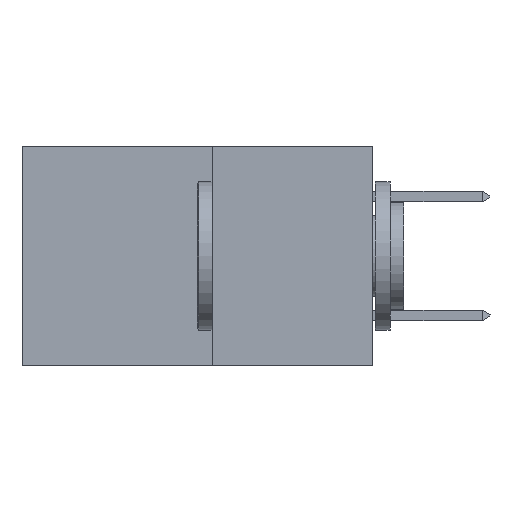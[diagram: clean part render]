
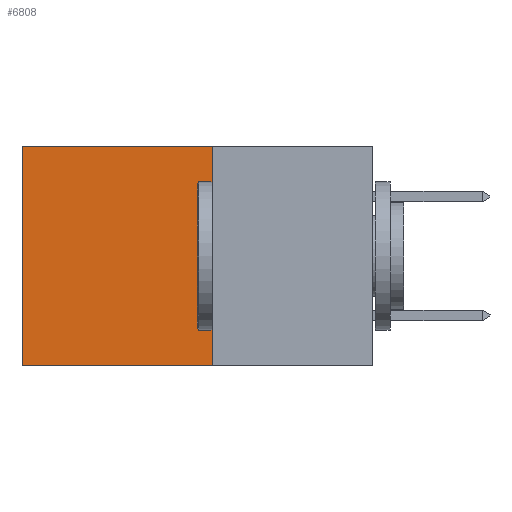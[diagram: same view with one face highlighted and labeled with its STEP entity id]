
A CAD part, left-side view. The second image highlights one B-rep face of the part: STEP entity #6808.
In plain terms, the highlighted planar face has unit normal (-1, 0, 0).
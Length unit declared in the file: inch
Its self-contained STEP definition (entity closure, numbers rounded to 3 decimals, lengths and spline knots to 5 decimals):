
#1793 = VERTEX_POINT ( 'NONE', #16363 ) ;
#2554 = ORIENTED_EDGE ( 'NONE', *, *, #5525, .T. ) ;
#2811 = EDGE_LOOP ( 'NONE', ( #19577, #14491, #19697, #2554 ) ) ;
#3418 = CARTESIAN_POINT ( 'NONE',  ( 0.277, 0.27, -0.37 ) ) ;
#3627 = DIRECTION ( 'NONE',  ( 0., 1., 0. ) ) ;
#3919 = VECTOR ( 'NONE', #4323, 39.37008 ) ;
#4057 = LINE ( 'NONE', #11294, #16284 ) ;
#4180 = VERTEX_POINT ( 'NONE', #18648 ) ;
#4323 = DIRECTION ( 'NONE',  ( 0., 0., -1. ) ) ;
#5525 = EDGE_CURVE ( 'NONE', #10825, #1793, #6654, .T. ) ;
#6654 = LINE ( 'NONE', #8165, #10359 ) ;
#6757 = EDGE_CURVE ( 'NONE', #10825, #4180, #4057, .T. ) ;
#6808 = ADVANCED_FACE ( 'NONE', ( #15302 ), #9431, .F. ) ;
#7058 = EDGE_CURVE ( 'NONE', #4180, #16475, #15545, .T. ) ;
#7857 = DIRECTION ( 'NONE',  ( 0., 1., 0. ) ) ;
#8104 = AXIS2_PLACEMENT_3D ( 'NONE', #9625, #9352, #9286 ) ;
#8165 = CARTESIAN_POINT ( 'NONE',  ( 0.277, 0.27, 0. ) ) ;
#8166 = LINE ( 'NONE', #12269, #3919 ) ;
#9286 = DIRECTION ( 'NONE',  ( 0., 0., -1. ) ) ;
#9352 = DIRECTION ( 'NONE',  ( 1., 0., 0. ) ) ;
#9431 = PLANE ( 'NONE',  #8104 ) ;
#9625 = CARTESIAN_POINT ( 'NONE',  ( 0.277, 0.27, -0.37 ) ) ;
#9941 = EDGE_CURVE ( 'NONE', #1793, #16475, #8166, .T. ) ;
#10308 = DIRECTION ( 'NONE',  ( 0., 0., -1. ) ) ;
#10359 = VECTOR ( 'NONE', #7857, 39.37008 ) ;
#10825 = VERTEX_POINT ( 'NONE', #14202 ) ;
#11294 = CARTESIAN_POINT ( 'NONE',  ( 0.277, 0.27, -0.37 ) ) ;
#11584 = CARTESIAN_POINT ( 'NONE',  ( 0.277, 0.59, -0.37 ) ) ;
#12269 = CARTESIAN_POINT ( 'NONE',  ( 0.277, 0.59, -0.37 ) ) ;
#14202 = CARTESIAN_POINT ( 'NONE',  ( 0.277, 0.27, 0. ) ) ;
#14491 = ORIENTED_EDGE ( 'NONE', *, *, #7058, .F. ) ;
#15302 = FACE_OUTER_BOUND ( 'NONE', #2811, .T. ) ;
#15545 = LINE ( 'NONE', #3418, #18662 ) ;
#16284 = VECTOR ( 'NONE', #10308, 39.37008 ) ;
#16363 = CARTESIAN_POINT ( 'NONE',  ( 0.277, 0.59, 0. ) ) ;
#16475 = VERTEX_POINT ( 'NONE', #11584 ) ;
#18648 = CARTESIAN_POINT ( 'NONE',  ( 0.277, 0.27, -0.37 ) ) ;
#18662 = VECTOR ( 'NONE', #3627, 39.37008 ) ;
#19577 = ORIENTED_EDGE ( 'NONE', *, *, #9941, .T. ) ;
#19697 = ORIENTED_EDGE ( 'NONE', *, *, #6757, .F. ) ;
